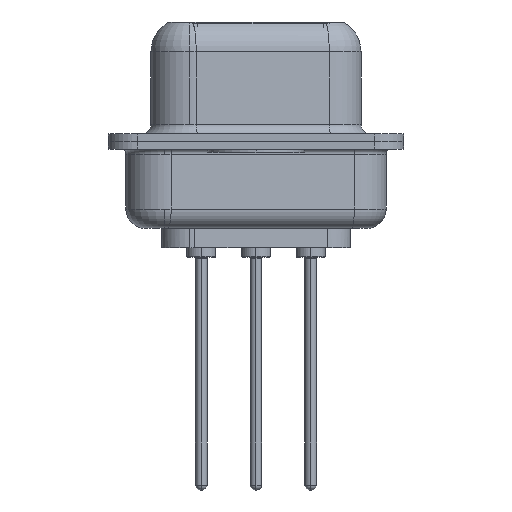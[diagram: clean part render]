
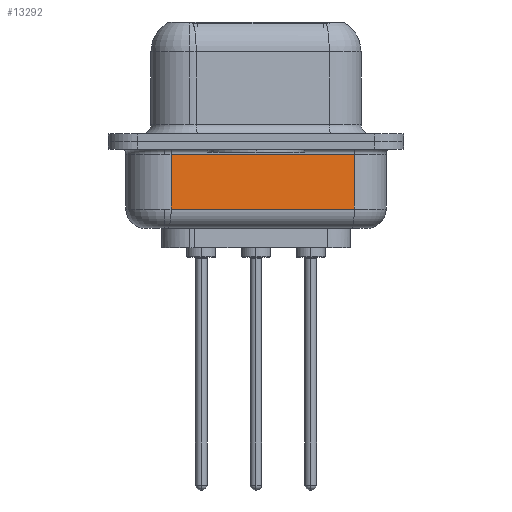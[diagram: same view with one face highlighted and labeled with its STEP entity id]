
A CAD part, left-side view. The second image highlights one B-rep face of the part: STEP entity #13292.
In plain terms, the highlighted planar face has unit normal (-0.985, -0.174, 0).
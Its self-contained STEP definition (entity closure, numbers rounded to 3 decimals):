
#163 = CARTESIAN_POINT ( 'NONE',  ( 4.605, -5.097, -0.65 ) ) ;
#166 = ORIENTED_EDGE ( 'NONE', *, *, #8765, .T. ) ;
#1122 = LINE ( 'NONE', #8354, #28613 ) ;
#1914 = CARTESIAN_POINT ( 'NONE',  ( 2.93, 4.403, -0.65 ) ) ;
#2318 = FACE_OUTER_BOUND ( 'NONE', #30700, .T. ) ;
#2633 = DIRECTION ( 'NONE',  ( 0., 0., 1. ) ) ;
#2953 = DIRECTION ( 'NONE',  ( 0.985, 0.174, 0. ) ) ;
#4203 = CARTESIAN_POINT ( 'NONE',  ( 2.93, 4.403, -3.5 ) ) ;
#4354 = DIRECTION ( 'NONE',  ( 0.174, -0.985, 0. ) ) ;
#5145 = DIRECTION ( 'NONE',  ( -0.174, 0.985, 0. ) ) ;
#5559 = VERTEX_POINT ( 'NONE', #24894 ) ;
#5930 = LINE ( 'NONE', #4203, #19787 ) ;
#6790 = ORIENTED_EDGE ( 'NONE', *, *, #18376, .T. ) ;
#8354 = CARTESIAN_POINT ( 'NONE',  ( 2.93, 4.403, -4.5 ) ) ;
#8765 = EDGE_CURVE ( 'NONE', #11739, #5559, #30787, .T. ) ;
#10500 = ORIENTED_EDGE ( 'NONE', *, *, #25925, .T. ) ;
#11739 = VERTEX_POINT ( 'NONE', #163 ) ;
#11933 = LINE ( 'NONE', #19315, #27720 ) ;
#13292 = ADVANCED_FACE ( 'NONE', ( #2318 ), #28972, .F. ) ;
#13568 = DIRECTION ( 'NONE',  ( 0., 0., 1. ) ) ;
#13842 = ORIENTED_EDGE ( 'NONE', *, *, #17561, .F. ) ;
#16389 = VERTEX_POINT ( 'NONE', #25597 ) ;
#17375 = CARTESIAN_POINT ( 'NONE',  ( 2.93, 4.403, -3.5 ) ) ;
#17561 = EDGE_CURVE ( 'NONE', #24127, #5559, #1122, .T. ) ;
#18376 = EDGE_CURVE ( 'NONE', #16389, #11739, #11933, .T. ) ;
#18457 = AXIS2_PLACEMENT_3D ( 'NONE', #19476, #2953, #5145 ) ;
#19315 = CARTESIAN_POINT ( 'NONE',  ( 4.605, -5.097, -4.5 ) ) ;
#19476 = CARTESIAN_POINT ( 'NONE',  ( 2.93, 4.403, -4.5 ) ) ;
#19787 = VECTOR ( 'NONE', #4354, 1000. ) ;
#20519 = VECTOR ( 'NONE', #28266, 1000. ) ;
#24127 = VERTEX_POINT ( 'NONE', #17375 ) ;
#24894 = CARTESIAN_POINT ( 'NONE',  ( 2.93, 4.403, -0.65 ) ) ;
#25597 = CARTESIAN_POINT ( 'NONE',  ( 4.605, -5.097, -3.5 ) ) ;
#25925 = EDGE_CURVE ( 'NONE', #24127, #16389, #5930, .T. ) ;
#27720 = VECTOR ( 'NONE', #2633, 1000. ) ;
#28266 = DIRECTION ( 'NONE',  ( -0.174, 0.985, 0. ) ) ;
#28613 = VECTOR ( 'NONE', #13568, 1000. ) ;
#28972 = PLANE ( 'NONE',  #18457 ) ;
#30700 = EDGE_LOOP ( 'NONE', ( #13842, #10500, #6790, #166 ) ) ;
#30787 = LINE ( 'NONE', #1914, #20519 ) ;
